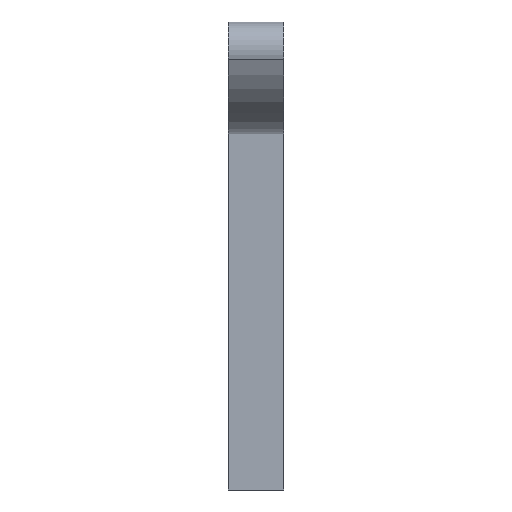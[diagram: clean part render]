
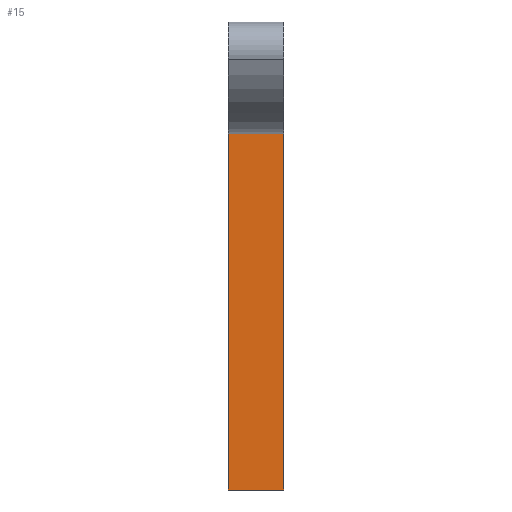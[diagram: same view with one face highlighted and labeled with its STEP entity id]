
A CAD part, front view. The second image highlights one B-rep face of the part: STEP entity #15.
In plain terms, the highlighted planar face has unit normal (0, -1, 0).
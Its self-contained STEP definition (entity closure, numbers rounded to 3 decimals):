
#7 = DIRECTION ( 'NONE',  ( 0., 0., -1. ) ) ;
#8 = EDGE_CURVE ( 'NONE', #624, #672, #594, .T. ) ;
#15 = ADVANCED_FACE ( 'NONE', ( #581 ), #526, .F. ) ;
#85 = CARTESIAN_POINT ( 'NONE',  ( 5., -5.181, -26.402 ) ) ;
#97 = CARTESIAN_POINT ( 'NONE',  ( 0., -5.181, -26.402 ) ) ;
#111 = ORIENTED_EDGE ( 'NONE', *, *, #136, .T. ) ;
#121 = DIRECTION ( 'NONE',  ( -1., 0., 0. ) ) ;
#123 = DIRECTION ( 'NONE',  ( 0., 0., -1. ) ) ;
#124 = CARTESIAN_POINT ( 'NONE',  ( 5., -5.181, 12.462 ) ) ;
#131 = EDGE_CURVE ( 'NONE', #672, #706, #470, .T. ) ;
#136 = EDGE_CURVE ( 'NONE', #624, #720, #469, .T. ) ;
#145 = CARTESIAN_POINT ( 'NONE',  ( 5., -5.181, 5.462 ) ) ;
#149 = CARTESIAN_POINT ( 'NONE',  ( 5., -5.181, -26.402 ) ) ;
#153 = CARTESIAN_POINT ( 'NONE',  ( 0., -5.181, 5.462 ) ) ;
#201 = EDGE_CURVE ( 'NONE', #706, #720, #431, .T. ) ;
#431 = LINE ( 'NONE', #85, #440 ) ;
#440 = VECTOR ( 'NONE', #121, 1000. ) ;
#461 = VECTOR ( 'NONE', #7, 1000. ) ;
#469 = LINE ( 'NONE', #853, #461 ) ;
#470 = LINE ( 'NONE', #124, #474 ) ;
#474 = VECTOR ( 'NONE', #123, 1000. ) ;
#526 = PLANE ( 'NONE',  #698 ) ;
#532 = DIRECTION ( 'NONE',  ( 0., 0., 1. ) ) ;
#576 = DIRECTION ( 'NONE',  ( 0., 1., 0. ) ) ;
#581 = FACE_OUTER_BOUND ( 'NONE', #832, .T. ) ;
#594 = LINE ( 'NONE', #833, #609 ) ;
#609 = VECTOR ( 'NONE', #779, 1000. ) ;
#624 = VERTEX_POINT ( 'NONE', #153 ) ;
#672 = VERTEX_POINT ( 'NONE', #145 ) ;
#691 = CARTESIAN_POINT ( 'NONE',  ( 5., -5.181, 12.462 ) ) ;
#698 = AXIS2_PLACEMENT_3D ( 'NONE', #691, #576, #532 ) ;
#702 = ORIENTED_EDGE ( 'NONE', *, *, #131, .F. ) ;
#706 = VERTEX_POINT ( 'NONE', #149 ) ;
#720 = VERTEX_POINT ( 'NONE', #97 ) ;
#730 = ORIENTED_EDGE ( 'NONE', *, *, #8, .F. ) ;
#740 = ORIENTED_EDGE ( 'NONE', *, *, #201, .F. ) ;
#779 = DIRECTION ( 'NONE',  ( 1., 0., 0. ) ) ;
#832 = EDGE_LOOP ( 'NONE', ( #730, #111, #740, #702 ) ) ;
#833 = CARTESIAN_POINT ( 'NONE',  ( 5., -5.181, 5.462 ) ) ;
#853 = CARTESIAN_POINT ( 'NONE',  ( 0., -5.181, 12.462 ) ) ;
